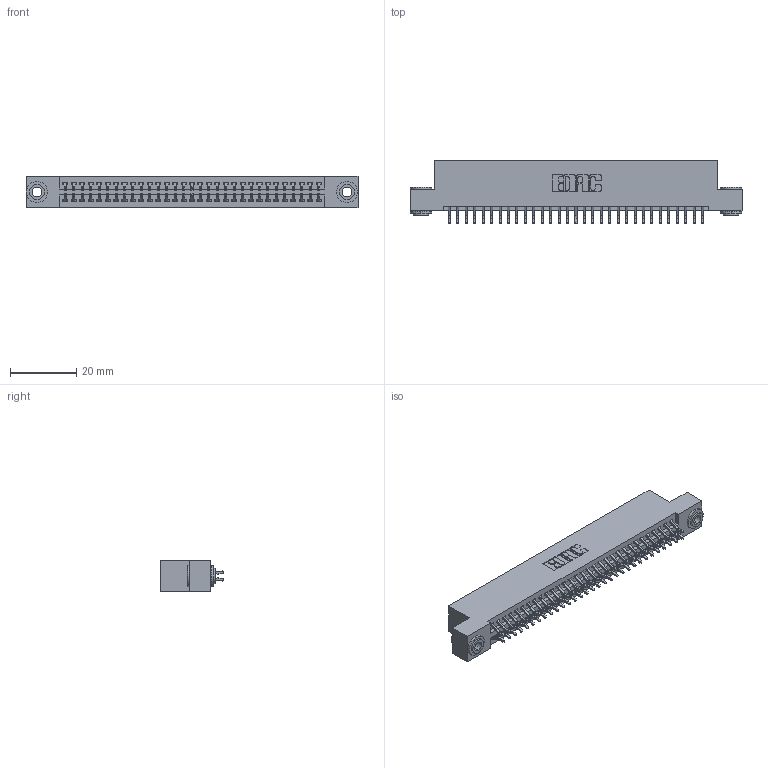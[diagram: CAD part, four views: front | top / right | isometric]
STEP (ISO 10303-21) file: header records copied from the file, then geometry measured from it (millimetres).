
FILE_DESCRIPTION (( 'STEP AP203' ), '1' );
FILE_NAME ('345-062-556-203.STEP', '2019-10-30T12:09:25', ( '' ), ( '' ), 'SwSTEP 2.0', 'SolidWorks 2016', '' );
FILE_SCHEMA (( 'CONFIG_CONTROL_DESIGN' ));
Length unit declared in the file: inch
Products named in the file (4): 345-062-556-203; 345 Part_Flush Mounting Lugs - 0.156 Dia-TH; 345-292-001_556 Tail; 345-250-002_345-250-002-102
Assembly tree (65 placements, depth 2):
  345-062-556-203
    345 Part_Flush Mounting Lugs - 0.156 Dia-TH
    345-292-001_556 Tail  x62
    345-250-002_345-250-002-102  x2
Bounding box: 99.95 x 19.24 x 9.4 mm (x, y, z)
Volume: 9624 mm3; surface area: 14163.4 mm2
Topology: 65 solids, 65 shells, 3636 faces, 10771 edges, 7094 vertices
Faces by surface type: plane 2384, cylinder 1244, cone 8
Entity records: 26674 total; most frequent: CARTESIAN_POINT 4471, ORIENTED_EDGE 4386, DIRECTION 3975, EDGE_CURVE 2193, VECTOR 1905, LINE 1905, VERTEX_POINT 1458, AXIS2_PLACEMENT_3D 1035
